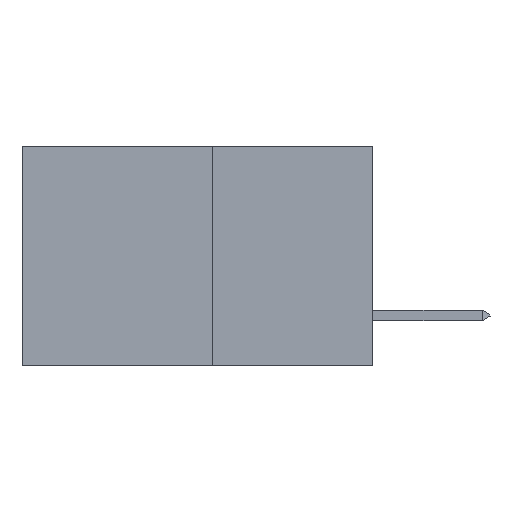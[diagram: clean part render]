
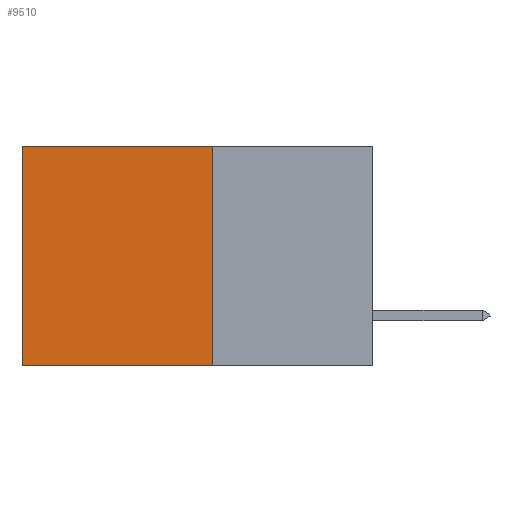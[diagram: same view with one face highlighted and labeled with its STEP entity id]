
A CAD part, left-side view. The second image highlights one B-rep face of the part: STEP entity #9510.
In plain terms, the highlighted planar face has unit normal (-1, 0, 0).
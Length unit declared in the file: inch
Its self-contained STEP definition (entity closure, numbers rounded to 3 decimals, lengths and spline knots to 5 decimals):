
#194 = DIRECTION ( 'NONE',  ( 0., 0., -1. ) ) ;
#1350 = VECTOR ( 'NONE', #15451, 39.37008 ) ;
#1381 = LINE ( 'NONE', #5116, #15826 ) ;
#1956 = EDGE_CURVE ( 'NONE', #12867, #14527, #1381, .T. ) ;
#2825 = EDGE_CURVE ( 'NONE', #7268, #14527, #12513, .T. ) ;
#3137 = LINE ( 'NONE', #8693, #10665 ) ;
#3694 = ORIENTED_EDGE ( 'NONE', *, *, #5211, .T. ) ;
#3922 = CARTESIAN_POINT ( 'NONE',  ( 0.277, 0.59, -0.37 ) ) ;
#4162 = DIRECTION ( 'NONE',  ( 0., 1., 0. ) ) ;
#4185 = CARTESIAN_POINT ( 'NONE',  ( 0.277, 0.27, 0. ) ) ;
#5116 = CARTESIAN_POINT ( 'NONE',  ( 0.277, 0.27, -0.37 ) ) ;
#5211 = EDGE_CURVE ( 'NONE', #7341, #7268, #12352, .T. ) ;
#6550 = PLANE ( 'NONE',  #11960 ) ;
#6878 = ORIENTED_EDGE ( 'NONE', *, *, #1956, .F. ) ;
#7268 = VERTEX_POINT ( 'NONE', #8719 ) ;
#7341 = VERTEX_POINT ( 'NONE', #17107 ) ;
#7989 = DIRECTION ( 'NONE',  ( 1., 0., 0. ) ) ;
#8693 = CARTESIAN_POINT ( 'NONE',  ( 0.277, 0.27, -0.37 ) ) ;
#8719 = CARTESIAN_POINT ( 'NONE',  ( 0.277, 0.59, 0. ) ) ;
#9510 = ADVANCED_FACE ( 'NONE', ( #14616 ), #6550, .F. ) ;
#10665 = VECTOR ( 'NONE', #194, 39.37008 ) ;
#11195 = ORIENTED_EDGE ( 'NONE', *, *, #17927, .F. ) ;
#11919 = VECTOR ( 'NONE', #4162, 39.37008 ) ;
#11960 = AXIS2_PLACEMENT_3D ( 'NONE', #16275, #7989, #17639 ) ;
#12352 = LINE ( 'NONE', #4185, #11919 ) ;
#12513 = LINE ( 'NONE', #3922, #1350 ) ;
#12748 = DIRECTION ( 'NONE',  ( 0., 1., 0. ) ) ;
#12867 = VERTEX_POINT ( 'NONE', #16128 ) ;
#12991 = CARTESIAN_POINT ( 'NONE',  ( 0.277, 0.59, -0.37 ) ) ;
#14527 = VERTEX_POINT ( 'NONE', #12991 ) ;
#14616 = FACE_OUTER_BOUND ( 'NONE', #15186, .T. ) ;
#15186 = EDGE_LOOP ( 'NONE', ( #15310, #6878, #11195, #3694 ) ) ;
#15310 = ORIENTED_EDGE ( 'NONE', *, *, #2825, .T. ) ;
#15451 = DIRECTION ( 'NONE',  ( 0., 0., -1. ) ) ;
#15826 = VECTOR ( 'NONE', #12748, 39.37008 ) ;
#16128 = CARTESIAN_POINT ( 'NONE',  ( 0.277, 0.27, -0.37 ) ) ;
#16275 = CARTESIAN_POINT ( 'NONE',  ( 0.277, 0.27, -0.37 ) ) ;
#17107 = CARTESIAN_POINT ( 'NONE',  ( 0.277, 0.27, 0. ) ) ;
#17639 = DIRECTION ( 'NONE',  ( 0., 0., -1. ) ) ;
#17927 = EDGE_CURVE ( 'NONE', #7341, #12867, #3137, .T. ) ;
